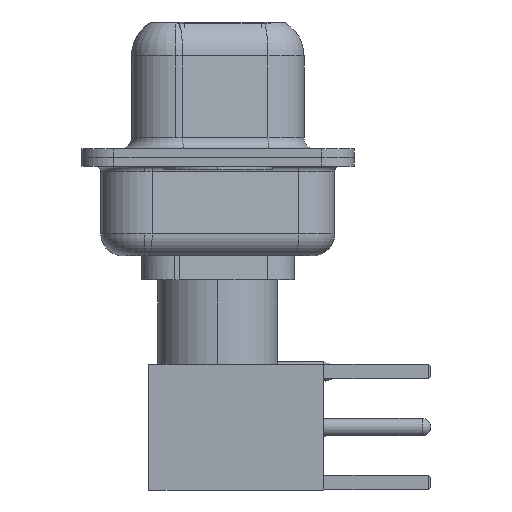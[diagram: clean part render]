
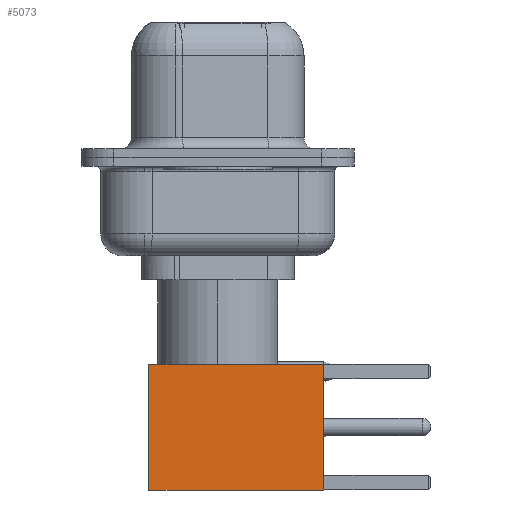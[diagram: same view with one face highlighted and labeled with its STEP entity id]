
A CAD part, left-side view. The second image highlights one B-rep face of the part: STEP entity #5073.
In plain terms, the highlighted face is planar.
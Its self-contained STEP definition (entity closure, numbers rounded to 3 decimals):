
#695 = CARTESIAN_POINT ( 'NONE',  ( 2.875, 2.875, 0. ) ) ;
#1415 = VECTOR ( 'NONE', #14443, 1000. ) ;
#1868 = DIRECTION ( 'NONE',  ( -1., 0., 0. ) ) ;
#3740 = CARTESIAN_POINT ( 'NONE',  ( -2.875, 2.875, 0. ) ) ;
#3789 = LINE ( 'NONE', #17814, #15972 ) ;
#3798 = VERTEX_POINT ( 'NONE', #19709 ) ;
#4522 = VECTOR ( 'NONE', #21129, 1000. ) ;
#4840 = CARTESIAN_POINT ( 'NONE',  ( 2.875, 2.875, 0. ) ) ;
#4911 = EDGE_CURVE ( 'NONE', #14813, #3798, #6404, .T. ) ;
#4915 = CARTESIAN_POINT ( 'NONE',  ( 0., 2.875, 8. ) ) ;
#5024 = DIRECTION ( 'NONE',  ( -1., 0., 0. ) ) ;
#5073 = ADVANCED_FACE ( 'NONE', ( #15957 ), #5262, .T. ) ;
#5262 = PLANE ( 'NONE',  #20802 ) ;
#5600 = DIRECTION ( 'NONE',  ( 0., 1., 0. ) ) ;
#5639 = LINE ( 'NONE', #16221, #4522 ) ;
#6404 = LINE ( 'NONE', #4915, #17888 ) ;
#6940 = EDGE_CURVE ( 'NONE', #3798, #14628, #7416, .T. ) ;
#7416 = LINE ( 'NONE', #3740, #1415 ) ;
#10873 = ORIENTED_EDGE ( 'NONE', *, *, #20751, .T. ) ;
#13027 = CARTESIAN_POINT ( 'NONE',  ( 2.875, 2.875, 8. ) ) ;
#13580 = ORIENTED_EDGE ( 'NONE', *, *, #22074, .T. ) ;
#14443 = DIRECTION ( 'NONE',  ( 0., 0., -1. ) ) ;
#14628 = VERTEX_POINT ( 'NONE', #15690 ) ;
#14813 = VERTEX_POINT ( 'NONE', #13027 ) ;
#15668 = ORIENTED_EDGE ( 'NONE', *, *, #6940, .F. ) ;
#15690 = CARTESIAN_POINT ( 'NONE',  ( -2.875, 2.875, 0. ) ) ;
#15957 = FACE_OUTER_BOUND ( 'NONE', #20060, .T. ) ;
#15972 = VECTOR ( 'NONE', #1868, 1000. ) ;
#16221 = CARTESIAN_POINT ( 'NONE',  ( 2.875, 2.875, 0. ) ) ;
#17814 = CARTESIAN_POINT ( 'NONE',  ( 0., 2.875, 0. ) ) ;
#17888 = VECTOR ( 'NONE', #5024, 1000. ) ;
#18836 = VERTEX_POINT ( 'NONE', #695 ) ;
#19709 = CARTESIAN_POINT ( 'NONE',  ( -2.875, 2.875, 8. ) ) ;
#20060 = EDGE_LOOP ( 'NONE', ( #10873, #13580, #15668, #21146 ) ) ;
#20751 = EDGE_CURVE ( 'NONE', #14813, #18836, #5639, .T. ) ;
#20802 = AXIS2_PLACEMENT_3D ( 'NONE', #4840, #5600, #20987 ) ;
#20987 = DIRECTION ( 'NONE',  ( 0., 0., 1. ) ) ;
#21129 = DIRECTION ( 'NONE',  ( 0., 0., -1. ) ) ;
#21146 = ORIENTED_EDGE ( 'NONE', *, *, #4911, .F. ) ;
#22074 = EDGE_CURVE ( 'NONE', #18836, #14628, #3789, .T. ) ;
